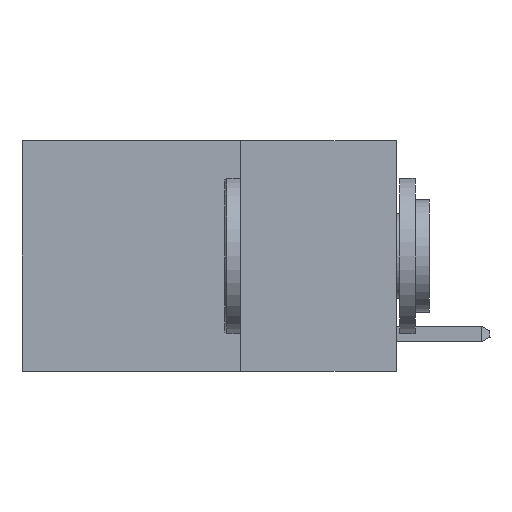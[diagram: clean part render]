
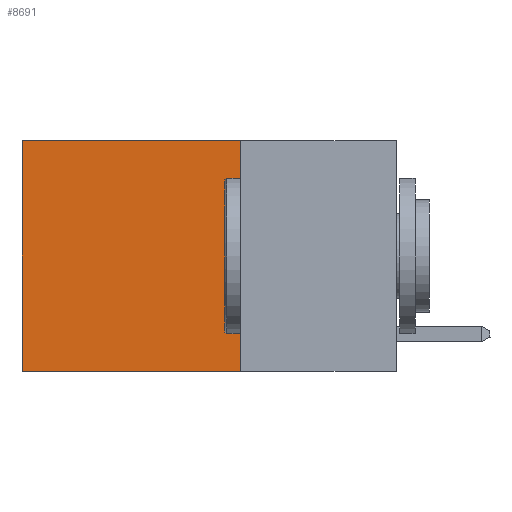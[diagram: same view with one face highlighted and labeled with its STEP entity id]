
A CAD part, left-side view. The second image highlights one B-rep face of the part: STEP entity #8691.
In plain terms, the highlighted planar face has unit normal (-1, 0, 0).
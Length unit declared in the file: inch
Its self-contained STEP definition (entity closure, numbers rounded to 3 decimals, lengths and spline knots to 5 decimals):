
#29 = ORIENTED_EDGE ( 'NONE', *, *, #8743, .F. ) ;
#621 = DIRECTION ( 'NONE',  ( 1., 0., 0. ) ) ;
#756 = CARTESIAN_POINT ( 'NONE',  ( 0.2625, 0.6, -0.37 ) ) ;
#774 = LINE ( 'NONE', #2408, #4523 ) ;
#1489 = CARTESIAN_POINT ( 'NONE',  ( 0.2625, 0.6, 0. ) ) ;
#1728 = ORIENTED_EDGE ( 'NONE', *, *, #18151, .T. ) ;
#2408 = CARTESIAN_POINT ( 'NONE',  ( 0.2625, 0.25, 0. ) ) ;
#2476 = CARTESIAN_POINT ( 'NONE',  ( 0.2625, 0.25, -0.37 ) ) ;
#2704 = DIRECTION ( 'NONE',  ( 0., 0., -1. ) ) ;
#2787 = EDGE_CURVE ( 'NONE', #7612, #19200, #20748, .T. ) ;
#3324 = VECTOR ( 'NONE', #9525, 39.37008 ) ;
#3410 = ORIENTED_EDGE ( 'NONE', *, *, #5138, .F. ) ;
#3632 = ORIENTED_EDGE ( 'NONE', *, *, #2787, .T. ) ;
#4523 = VECTOR ( 'NONE', #14510, 39.37008 ) ;
#5138 = EDGE_CURVE ( 'NONE', #11245, #6841, #15997, .T. ) ;
#5946 = PLANE ( 'NONE',  #6610 ) ;
#6078 = VECTOR ( 'NONE', #8726, 39.37008 ) ;
#6106 = EDGE_LOOP ( 'NONE', ( #3632, #29, #3410, #1728 ) ) ;
#6610 = AXIS2_PLACEMENT_3D ( 'NONE', #18053, #621, #2704 ) ;
#6841 = VERTEX_POINT ( 'NONE', #19545 ) ;
#7612 = VERTEX_POINT ( 'NONE', #20199 ) ;
#8691 = ADVANCED_FACE ( 'NONE', ( #11032 ), #5946, .F. ) ;
#8726 = DIRECTION ( 'NONE',  ( 0., 0., -1. ) ) ;
#8743 = EDGE_CURVE ( 'NONE', #6841, #19200, #11478, .T. ) ;
#8768 = CARTESIAN_POINT ( 'NONE',  ( 0.2625, 0.25, 0. ) ) ;
#9525 = DIRECTION ( 'NONE',  ( 0., 1., 0. ) ) ;
#11032 = FACE_OUTER_BOUND ( 'NONE', #6106, .T. ) ;
#11245 = VERTEX_POINT ( 'NONE', #8768 ) ;
#11478 = LINE ( 'NONE', #2476, #3324 ) ;
#12544 = CARTESIAN_POINT ( 'NONE',  ( 0.2625, 0.25, 0. ) ) ;
#13527 = VECTOR ( 'NONE', #15345, 39.37008 ) ;
#14510 = DIRECTION ( 'NONE',  ( 0., 1., 0. ) ) ;
#15345 = DIRECTION ( 'NONE',  ( 0., 0., -1. ) ) ;
#15997 = LINE ( 'NONE', #12544, #6078 ) ;
#18053 = CARTESIAN_POINT ( 'NONE',  ( 0.2625, 0.25, 0. ) ) ;
#18151 = EDGE_CURVE ( 'NONE', #11245, #7612, #774, .T. ) ;
#19200 = VERTEX_POINT ( 'NONE', #756 ) ;
#19545 = CARTESIAN_POINT ( 'NONE',  ( 0.2625, 0.25, -0.37 ) ) ;
#20199 = CARTESIAN_POINT ( 'NONE',  ( 0.2625, 0.6, 0. ) ) ;
#20748 = LINE ( 'NONE', #1489, #13527 ) ;
